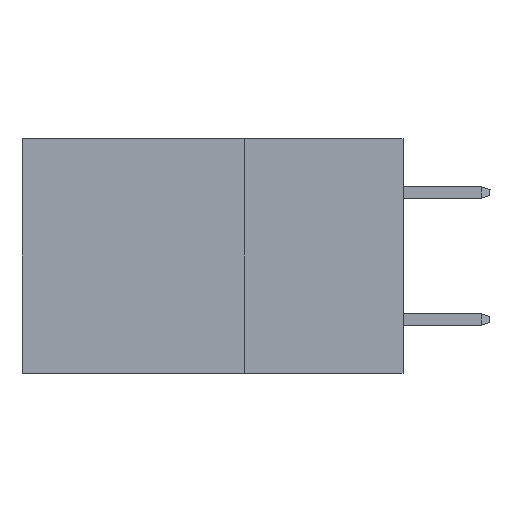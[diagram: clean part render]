
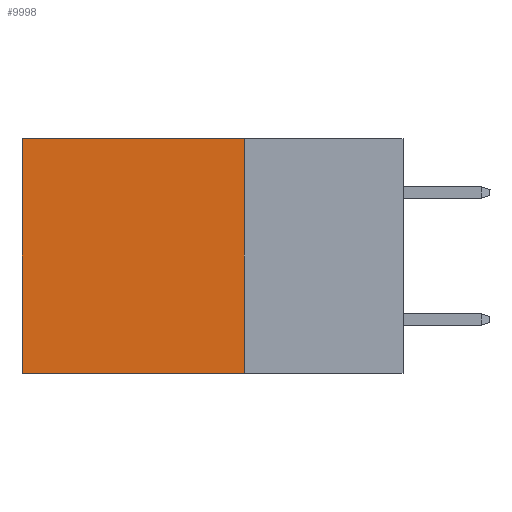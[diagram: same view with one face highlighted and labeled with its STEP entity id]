
A CAD part, left-side view. The second image highlights one B-rep face of the part: STEP entity #9998.
In plain terms, the highlighted planar face has unit normal (-1, 0, 0).
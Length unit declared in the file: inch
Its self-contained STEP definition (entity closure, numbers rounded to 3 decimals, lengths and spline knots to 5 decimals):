
#488 = DIRECTION ( 'NONE',  ( 1., 0., 0. ) ) ;
#787 = PLANE ( 'NONE',  #2307 ) ;
#2307 = AXIS2_PLACEMENT_3D ( 'NONE', #17312, #488, #20345 ) ;
#3499 = EDGE_CURVE ( 'NONE', #29946, #19664, #4136, .T. ) ;
#4136 = LINE ( 'NONE', #18548, #7065 ) ;
#5568 = EDGE_LOOP ( 'NONE', ( #17095, #9150, #17431, #14379 ) ) ;
#6474 = CARTESIAN_POINT ( 'NONE',  ( 0.2875, 0.25, 0. ) ) ;
#7065 = VECTOR ( 'NONE', #8929, 39.37008 ) ;
#8024 = VECTOR ( 'NONE', #23707, 39.37008 ) ;
#8882 = CARTESIAN_POINT ( 'NONE',  ( 0.2875, 0.25, -0.37 ) ) ;
#8929 = DIRECTION ( 'NONE',  ( 0., 1., 0. ) ) ;
#9150 = ORIENTED_EDGE ( 'NONE', *, *, #3499, .F. ) ;
#9700 = DIRECTION ( 'NONE',  ( 0., 0., -1. ) ) ;
#9998 = ADVANCED_FACE ( 'NONE', ( #17617 ), #787, .F. ) ;
#10183 = LINE ( 'NONE', #26876, #16751 ) ;
#11316 = EDGE_CURVE ( 'NONE', #18308, #28316, #17501, .T. ) ;
#14379 = ORIENTED_EDGE ( 'NONE', *, *, #11316, .T. ) ;
#15464 = CARTESIAN_POINT ( 'NONE',  ( 0.2875, 0.6, 0. ) ) ;
#16751 = VECTOR ( 'NONE', #9700, 39.37008 ) ;
#17095 = ORIENTED_EDGE ( 'NONE', *, *, #30983, .T. ) ;
#17312 = CARTESIAN_POINT ( 'NONE',  ( 0.2875, 0.25, 0. ) ) ;
#17431 = ORIENTED_EDGE ( 'NONE', *, *, #21151, .F. ) ;
#17501 = LINE ( 'NONE', #19595, #31562 ) ;
#17617 = FACE_OUTER_BOUND ( 'NONE', #5568, .T. ) ;
#18308 = VERTEX_POINT ( 'NONE', #6474 ) ;
#18548 = CARTESIAN_POINT ( 'NONE',  ( 0.2875, 0.25, -0.37 ) ) ;
#18704 = CARTESIAN_POINT ( 'NONE',  ( 0.2875, 0.25, 0. ) ) ;
#19595 = CARTESIAN_POINT ( 'NONE',  ( 0.2875, 0.25, 0. ) ) ;
#19664 = VERTEX_POINT ( 'NONE', #27696 ) ;
#20345 = DIRECTION ( 'NONE',  ( 0., 0., -1. ) ) ;
#21151 = EDGE_CURVE ( 'NONE', #18308, #29946, #30882, .T. ) ;
#21863 = DIRECTION ( 'NONE',  ( 0., 1., 0. ) ) ;
#23707 = DIRECTION ( 'NONE',  ( 0., 0., -1. ) ) ;
#26876 = CARTESIAN_POINT ( 'NONE',  ( 0.2875, 0.6, 0. ) ) ;
#27696 = CARTESIAN_POINT ( 'NONE',  ( 0.2875, 0.6, -0.37 ) ) ;
#28316 = VERTEX_POINT ( 'NONE', #15464 ) ;
#29946 = VERTEX_POINT ( 'NONE', #8882 ) ;
#30882 = LINE ( 'NONE', #18704, #8024 ) ;
#30983 = EDGE_CURVE ( 'NONE', #28316, #19664, #10183, .T. ) ;
#31562 = VECTOR ( 'NONE', #21863, 39.37008 ) ;
